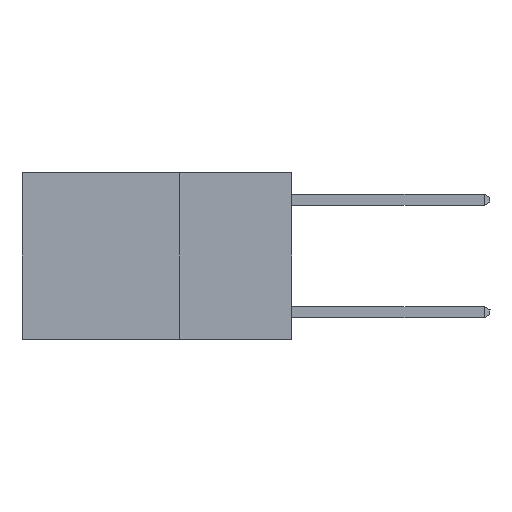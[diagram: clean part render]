
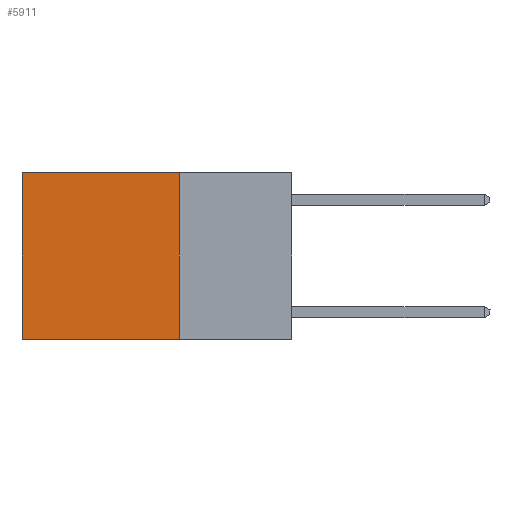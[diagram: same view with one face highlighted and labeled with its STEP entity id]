
A CAD part, left-side view. The second image highlights one B-rep face of the part: STEP entity #5911.
In plain terms, the highlighted planar face has unit normal (-1, 0, 0).
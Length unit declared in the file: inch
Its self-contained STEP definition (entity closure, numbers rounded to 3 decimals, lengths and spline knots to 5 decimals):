
#338 = VECTOR ( 'NONE', #2971, 39.37008 ) ;
#508 = EDGE_CURVE ( 'NONE', #9482, #926, #7124, .T. ) ;
#631 = DIRECTION ( 'NONE',  ( 0., 1., 0. ) ) ;
#838 = PLANE ( 'NONE',  #1827 ) ;
#926 = VERTEX_POINT ( 'NONE', #4789 ) ;
#959 = ORIENTED_EDGE ( 'NONE', *, *, #4960, .T. ) ;
#973 = ORIENTED_EDGE ( 'NONE', *, *, #8402, .F. ) ;
#996 = ORIENTED_EDGE ( 'NONE', *, *, #6489, .F. ) ;
#1027 = ORIENTED_EDGE ( 'NONE', *, *, #508, .T. ) ;
#1321 = CARTESIAN_POINT ( 'NONE',  ( 0.2625, 0.25, -0.37 ) ) ;
#1549 = LINE ( 'NONE', #8526, #9727 ) ;
#1725 = CARTESIAN_POINT ( 'NONE',  ( 0.2625, 0.25, 0. ) ) ;
#1741 = DIRECTION ( 'NONE',  ( 1., 0., 0. ) ) ;
#1827 = AXIS2_PLACEMENT_3D ( 'NONE', #6524, #1741, #7265 ) ;
#2147 = CARTESIAN_POINT ( 'NONE',  ( 0.2625, 0.6, 0. ) ) ;
#2703 = LINE ( 'NONE', #2147, #338 ) ;
#2889 = CARTESIAN_POINT ( 'NONE',  ( 0.2625, 0.25, 0. ) ) ;
#2971 = DIRECTION ( 'NONE',  ( 0., 0., -1. ) ) ;
#3367 = VECTOR ( 'NONE', #10116, 39.37008 ) ;
#4163 = DIRECTION ( 'NONE',  ( 0., 1., 0. ) ) ;
#4703 = VERTEX_POINT ( 'NONE', #4978 ) ;
#4789 = CARTESIAN_POINT ( 'NONE',  ( 0.2625, 0.6, 0. ) ) ;
#4960 = EDGE_CURVE ( 'NONE', #926, #4703, #2703, .T. ) ;
#4978 = CARTESIAN_POINT ( 'NONE',  ( 0.2625, 0.6, -0.37 ) ) ;
#5063 = VECTOR ( 'NONE', #4163, 39.37008 ) ;
#5911 = ADVANCED_FACE ( 'NONE', ( #7166 ), #838, .F. ) ;
#6489 = EDGE_CURVE ( 'NONE', #9482, #8943, #9402, .T. ) ;
#6524 = CARTESIAN_POINT ( 'NONE',  ( 0.2625, 0.25, 0. ) ) ;
#6536 = CARTESIAN_POINT ( 'NONE',  ( 0.2625, 0.25, 0. ) ) ;
#7124 = LINE ( 'NONE', #6536, #5063 ) ;
#7166 = FACE_OUTER_BOUND ( 'NONE', #10155, .T. ) ;
#7265 = DIRECTION ( 'NONE',  ( 0., 0., -1. ) ) ;
#8402 = EDGE_CURVE ( 'NONE', #8943, #4703, #1549, .T. ) ;
#8526 = CARTESIAN_POINT ( 'NONE',  ( 0.2625, 0.25, -0.37 ) ) ;
#8943 = VERTEX_POINT ( 'NONE', #1321 ) ;
#9402 = LINE ( 'NONE', #1725, #3367 ) ;
#9482 = VERTEX_POINT ( 'NONE', #2889 ) ;
#9727 = VECTOR ( 'NONE', #631, 39.37008 ) ;
#10116 = DIRECTION ( 'NONE',  ( 0., 0., -1. ) ) ;
#10155 = EDGE_LOOP ( 'NONE', ( #959, #973, #996, #1027 ) ) ;
